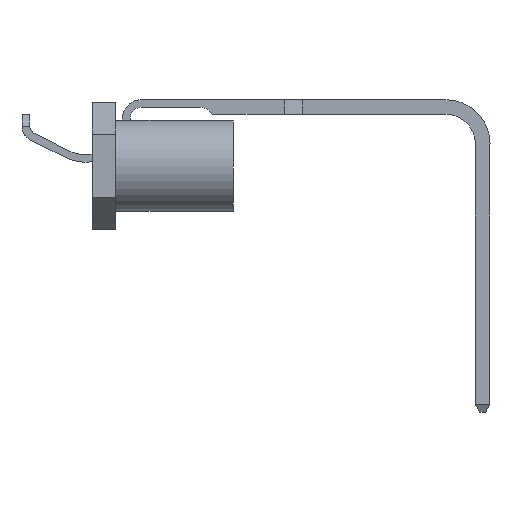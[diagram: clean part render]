
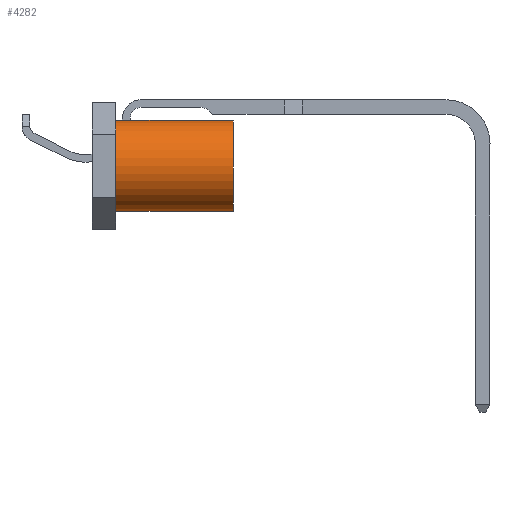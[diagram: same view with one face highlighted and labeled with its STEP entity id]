
A CAD part, left-side view. The second image highlights one B-rep face of the part: STEP entity #4282.
In plain terms, the highlighted cylindrical face has radius 1.968 mm (diameter 3.937 mm), a partial arc.
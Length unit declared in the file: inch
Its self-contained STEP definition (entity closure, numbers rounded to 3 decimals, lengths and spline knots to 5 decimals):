
#439 = CARTESIAN_POINT ( 'NONE',  ( 0., 0.04, -0.0775 ) ) ;
#582 = EDGE_CURVE ( 'NONE', #769, #6501, #16042, .T. ) ;
#769 = VERTEX_POINT ( 'NONE', #439 ) ;
#1243 = DIRECTION ( 'NONE',  ( 0., -1., 0. ) ) ;
#1803 = EDGE_CURVE ( 'NONE', #19415, #6501, #10391, .T. ) ;
#2247 = CYLINDRICAL_SURFACE ( 'NONE', #11943, 0.0775 ) ;
#2696 = AXIS2_PLACEMENT_3D ( 'NONE', #19139, #8791, #13714 ) ;
#3407 = DIRECTION ( 'NONE',  ( 0., 1., 0. ) ) ;
#3449 = ORIENTED_EDGE ( 'NONE', *, *, #582, .T. ) ;
#3533 = CARTESIAN_POINT ( 'NONE',  ( 0., 0.24, -0.0775 ) ) ;
#3883 = EDGE_CURVE ( 'NONE', #8450, #769, #9565, .T. ) ;
#4282 = ADVANCED_FACE ( 'NONE', ( #10529 ), #2247, .T. ) ;
#5077 = AXIS2_PLACEMENT_3D ( 'NONE', #12624, #3407, #14172 ) ;
#5099 = DIRECTION ( 'NONE',  ( 0., -1., 0. ) ) ;
#5959 = DIRECTION ( 'NONE',  ( 0., 0., -1. ) ) ;
#6149 = ORIENTED_EDGE ( 'NONE', *, *, #1803, .F. ) ;
#6501 = VERTEX_POINT ( 'NONE', #12307 ) ;
#6622 = EDGE_CURVE ( 'NONE', #8450, #19415, #13783, .T. ) ;
#7043 = CARTESIAN_POINT ( 'NONE',  ( 0., 0.24, -0.0775 ) ) ;
#8450 = VERTEX_POINT ( 'NONE', #7043 ) ;
#8471 = ORIENTED_EDGE ( 'NONE', *, *, #3883, .T. ) ;
#8791 = DIRECTION ( 'NONE',  ( 0., 1., 0. ) ) ;
#8927 = EDGE_LOOP ( 'NONE', ( #6149, #14251, #8471, #3449 ) ) ;
#9565 = LINE ( 'NONE', #3533, #14132 ) ;
#10391 = LINE ( 'NONE', #16544, #18006 ) ;
#10529 = FACE_OUTER_BOUND ( 'NONE', #8927, .T. ) ;
#11943 = AXIS2_PLACEMENT_3D ( 'NONE', #16657, #1243, #5959 ) ;
#12307 = CARTESIAN_POINT ( 'NONE',  ( 0., 0.04, 0.0775 ) ) ;
#12624 = CARTESIAN_POINT ( 'NONE',  ( 0., 0.24, 0. ) ) ;
#13714 = DIRECTION ( 'NONE',  ( 0., 0., 1. ) ) ;
#13783 = CIRCLE ( 'NONE', #5077, 0.0775 ) ;
#14132 = VECTOR ( 'NONE', #14297, 39.37008 ) ;
#14172 = DIRECTION ( 'NONE',  ( 0., 0., 1. ) ) ;
#14251 = ORIENTED_EDGE ( 'NONE', *, *, #6622, .F. ) ;
#14297 = DIRECTION ( 'NONE',  ( 0., -1., 0. ) ) ;
#16042 = CIRCLE ( 'NONE', #2696, 0.0775 ) ;
#16544 = CARTESIAN_POINT ( 'NONE',  ( 0., 0.24, 0.0775 ) ) ;
#16657 = CARTESIAN_POINT ( 'NONE',  ( 0., 0.24, 0. ) ) ;
#18006 = VECTOR ( 'NONE', #5099, 39.37008 ) ;
#19139 = CARTESIAN_POINT ( 'NONE',  ( 0., 0.04, 0. ) ) ;
#19415 = VERTEX_POINT ( 'NONE', #19439 ) ;
#19439 = CARTESIAN_POINT ( 'NONE',  ( 0., 0.24, 0.0775 ) ) ;
